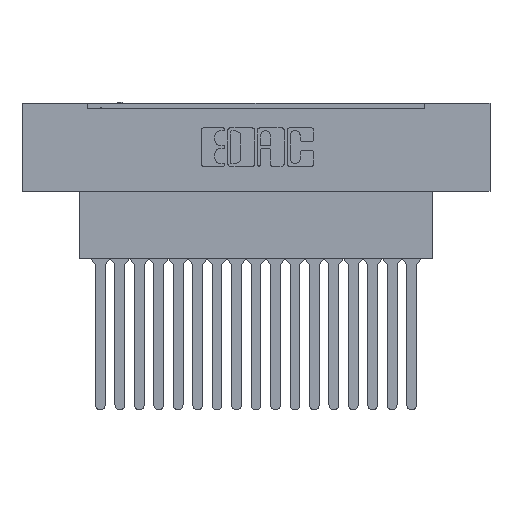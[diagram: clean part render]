
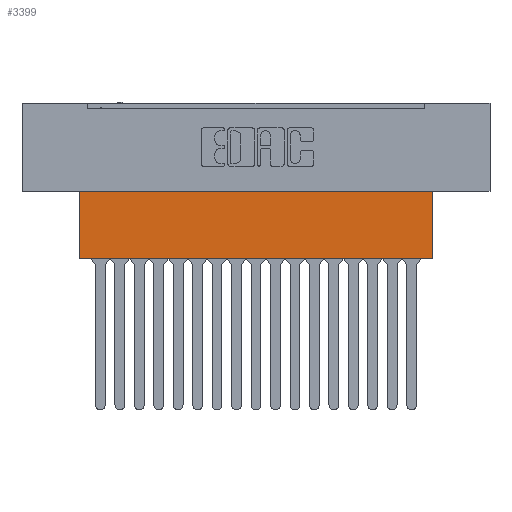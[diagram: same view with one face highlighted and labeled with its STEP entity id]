
A CAD part, top view. The second image highlights one B-rep face of the part: STEP entity #3399.
In plain terms, the highlighted planar face has unit normal (0, 0, 1).
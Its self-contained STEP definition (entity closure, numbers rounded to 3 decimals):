
#1611 = EDGE_CURVE ( 'NONE', #18486, #10989, #9293, .T. ) ;
#3193 = CARTESIAN_POINT ( 'NONE',  ( 7.468, -8.814, -3.962 ) ) ;
#3399 = ADVANCED_FACE ( 'NONE', ( #16085 ), #8460, .F. ) ;
#4129 = LINE ( 'NONE', #16257, #10200 ) ;
#4722 = CARTESIAN_POINT ( 'NONE',  ( 53.645, 0., -3.962 ) ) ;
#4947 = VECTOR ( 'NONE', #19744, 1000. ) ;
#5256 = EDGE_LOOP ( 'NONE', ( #10525, #18581, #13423, #23649 ) ) ;
#5414 = CARTESIAN_POINT ( 'NONE',  ( 61.112, 0., -3.962 ) ) ;
#5517 = CARTESIAN_POINT ( 'NONE',  ( 7.468, -8.814, -3.962 ) ) ;
#5788 = LINE ( 'NONE', #5414, #15560 ) ;
#5898 = EDGE_CURVE ( 'NONE', #10989, #14136, #4129, .T. ) ;
#6698 = VECTOR ( 'NONE', #18596, 1000. ) ;
#7161 = CARTESIAN_POINT ( 'NONE',  ( 7.468, 0., -3.962 ) ) ;
#7272 = DIRECTION ( 'NONE',  ( -1., 0., 0. ) ) ;
#7873 = EDGE_CURVE ( 'NONE', #18486, #21600, #5788, .T. ) ;
#8460 = PLANE ( 'NONE',  #11892 ) ;
#8606 = DIRECTION ( 'NONE',  ( 0., 0., -1. ) ) ;
#9293 = LINE ( 'NONE', #22410, #6698 ) ;
#10200 = VECTOR ( 'NONE', #11210, 1000. ) ;
#10525 = ORIENTED_EDGE ( 'NONE', *, *, #5898, .F. ) ;
#10639 = CARTESIAN_POINT ( 'NONE',  ( 53.645, -8.814, -3.962 ) ) ;
#10989 = VERTEX_POINT ( 'NONE', #10639 ) ;
#11210 = DIRECTION ( 'NONE',  ( -1., 0., 0. ) ) ;
#11892 = AXIS2_PLACEMENT_3D ( 'NONE', #21318, #8606, #15813 ) ;
#13423 = ORIENTED_EDGE ( 'NONE', *, *, #7873, .T. ) ;
#14136 = VERTEX_POINT ( 'NONE', #5517 ) ;
#15560 = VECTOR ( 'NONE', #7272, 1000. ) ;
#15813 = DIRECTION ( 'NONE',  ( 0., 1., 0. ) ) ;
#16085 = FACE_OUTER_BOUND ( 'NONE', #5256, .T. ) ;
#16257 = CARTESIAN_POINT ( 'NONE',  ( 61.112, -8.814, -3.962 ) ) ;
#17095 = EDGE_CURVE ( 'NONE', #14136, #21600, #23024, .T. ) ;
#18486 = VERTEX_POINT ( 'NONE', #4722 ) ;
#18581 = ORIENTED_EDGE ( 'NONE', *, *, #1611, .F. ) ;
#18596 = DIRECTION ( 'NONE',  ( 0., -1., 0. ) ) ;
#19744 = DIRECTION ( 'NONE',  ( 0., 1., 0. ) ) ;
#21318 = CARTESIAN_POINT ( 'NONE',  ( 61.112, 0., -3.962 ) ) ;
#21600 = VERTEX_POINT ( 'NONE', #7161 ) ;
#22410 = CARTESIAN_POINT ( 'NONE',  ( 53.645, -8.814, -3.962 ) ) ;
#23024 = LINE ( 'NONE', #3193, #4947 ) ;
#23649 = ORIENTED_EDGE ( 'NONE', *, *, #17095, .F. ) ;
